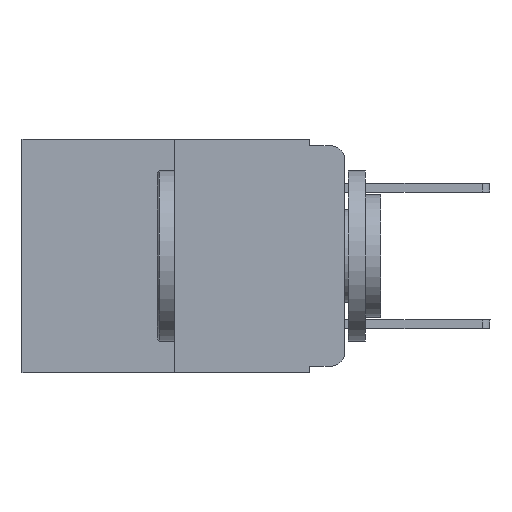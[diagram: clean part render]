
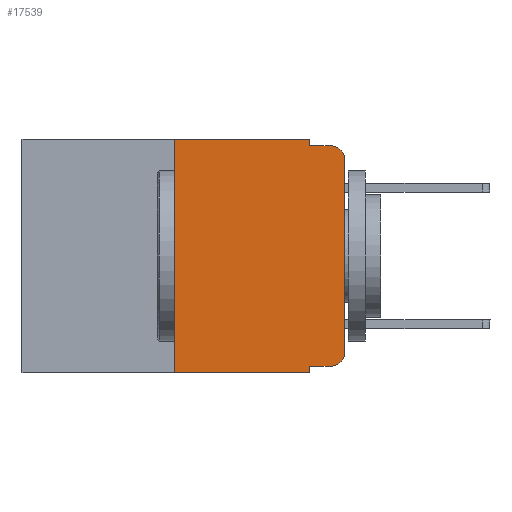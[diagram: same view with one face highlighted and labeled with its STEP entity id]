
A CAD part, left-side view. The second image highlights one B-rep face of the part: STEP entity #17539.
In plain terms, the highlighted planar face has unit normal (-1, 0, 0).
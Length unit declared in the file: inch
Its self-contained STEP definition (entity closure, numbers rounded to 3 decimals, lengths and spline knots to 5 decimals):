
#148 = DIRECTION ( 'NONE',  ( 0., 0., 1. ) ) ;
#819 = CARTESIAN_POINT ( 'NONE',  ( 0., 0.02, -0.333 ) ) ;
#824 = EDGE_CURVE ( 'NONE', #17543, #16498, #5310, .T. ) ;
#1425 = ORIENTED_EDGE ( 'NONE', *, *, #824, .T. ) ;
#1469 = CIRCLE ( 'NONE', #2114, 0.02 ) ;
#1476 = DIRECTION ( 'NONE',  ( 0., -1., 0. ) ) ;
#2114 = AXIS2_PLACEMENT_3D ( 'NONE', #15505, #2840, #5497 ) ;
#2137 = ORIENTED_EDGE ( 'NONE', *, *, #4531, .F. ) ;
#2203 = CARTESIAN_POINT ( 'NONE',  ( 0., 0.051, -0.01 ) ) ;
#2241 = VERTEX_POINT ( 'NONE', #5208 ) ;
#2840 = DIRECTION ( 'NONE',  ( -1., 0., 0. ) ) ;
#3317 = DIRECTION ( 'NONE',  ( 0., 0., -1. ) ) ;
#3366 = DIRECTION ( 'NONE',  ( 0., 0., 1. ) ) ;
#3472 = CARTESIAN_POINT ( 'NONE',  ( 0., 0.051, 0. ) ) ;
#3578 = VERTEX_POINT ( 'NONE', #6424 ) ;
#3598 = CARTESIAN_POINT ( 'NONE',  ( 0., 0.051, 0. ) ) ;
#3768 = VERTEX_POINT ( 'NONE', #4140 ) ;
#3793 = DIRECTION ( 'NONE',  ( 0., 0., -1. ) ) ;
#3851 = DIRECTION ( 'NONE',  ( 0., -1., 0. ) ) ;
#3922 = DIRECTION ( 'NONE',  ( 1., 0., 0. ) ) ;
#4140 = CARTESIAN_POINT ( 'NONE',  ( 0., 0.25, -0.343 ) ) ;
#4506 = VERTEX_POINT ( 'NONE', #819 ) ;
#4531 = EDGE_CURVE ( 'NONE', #5404, #17074, #15727, .T. ) ;
#4542 = CARTESIAN_POINT ( 'NONE',  ( 0., 0.02, -0.01 ) ) ;
#4837 = CIRCLE ( 'NONE', #16959, 0.02 ) ;
#5208 = CARTESIAN_POINT ( 'NONE',  ( 0., 0.051, 0. ) ) ;
#5210 = VECTOR ( 'NONE', #3851, 39.37008 ) ;
#5310 = LINE ( 'NONE', #6305, #10059 ) ;
#5404 = VERTEX_POINT ( 'NONE', #6133 ) ;
#5497 = DIRECTION ( 'NONE',  ( 0., 0., -1. ) ) ;
#5755 = ORIENTED_EDGE ( 'NONE', *, *, #17968, .T. ) ;
#5963 = EDGE_CURVE ( 'NONE', #3578, #2241, #13565, .T. ) ;
#6133 = CARTESIAN_POINT ( 'NONE',  ( 0., 0.051, -0.01 ) ) ;
#6236 = VECTOR ( 'NONE', #1476, 39.37008 ) ;
#6305 = CARTESIAN_POINT ( 'NONE',  ( 0., 0., 0. ) ) ;
#6424 = CARTESIAN_POINT ( 'NONE',  ( 0., 0.25, 0. ) ) ;
#6755 = VECTOR ( 'NONE', #13599, 39.37008 ) ;
#6838 = EDGE_CURVE ( 'NONE', #4506, #17543, #1469, .T. ) ;
#7303 = EDGE_CURVE ( 'NONE', #13460, #17790, #14835, .T. ) ;
#7308 = VECTOR ( 'NONE', #17732, 39.37008 ) ;
#7965 = ORIENTED_EDGE ( 'NONE', *, *, #7303, .F. ) ;
#9004 = CARTESIAN_POINT ( 'NONE',  ( 0., 0.051, -0.343 ) ) ;
#9016 = EDGE_CURVE ( 'NONE', #2241, #5404, #18085, .T. ) ;
#9068 = DIRECTION ( 'NONE',  ( 0., -1., 0. ) ) ;
#9200 = DIRECTION ( 'NONE',  ( -1., 0., 0. ) ) ;
#9745 = CARTESIAN_POINT ( 'NONE',  ( 0., 0., -0.03 ) ) ;
#9868 = CARTESIAN_POINT ( 'NONE',  ( 0., 0.051, -0.333 ) ) ;
#9935 = EDGE_LOOP ( 'NONE', ( #1425, #16983, #2137, #16027, #14566, #16875, #5755, #7965, #12602, #15670 ) ) ;
#10059 = VECTOR ( 'NONE', #3366, 39.37008 ) ;
#10118 = EDGE_CURVE ( 'NONE', #13460, #4506, #14705, .T. ) ;
#10657 = LINE ( 'NONE', #14892, #7308 ) ;
#10706 = DIRECTION ( 'NONE',  ( 0., 0., -1. ) ) ;
#11185 = LINE ( 'NONE', #11563, #12979 ) ;
#11563 = CARTESIAN_POINT ( 'NONE',  ( 0., 0.25, 0. ) ) ;
#12602 = ORIENTED_EDGE ( 'NONE', *, *, #10118, .T. ) ;
#12647 = FACE_OUTER_BOUND ( 'NONE', #9935, .T. ) ;
#12979 = VECTOR ( 'NONE', #148, 39.37008 ) ;
#13362 = CARTESIAN_POINT ( 'NONE',  ( 0., 0.02, -0.03 ) ) ;
#13460 = VERTEX_POINT ( 'NONE', #14985 ) ;
#13565 = LINE ( 'NONE', #14708, #16890 ) ;
#13599 = DIRECTION ( 'NONE',  ( 0., 0., -1. ) ) ;
#13761 = AXIS2_PLACEMENT_3D ( 'NONE', #16762, #3922, #3793 ) ;
#14152 = EDGE_CURVE ( 'NONE', #3768, #3578, #11185, .T. ) ;
#14566 = ORIENTED_EDGE ( 'NONE', *, *, #5963, .F. ) ;
#14705 = LINE ( 'NONE', #9868, #6236 ) ;
#14708 = CARTESIAN_POINT ( 'NONE',  ( 0., 0.473, 0. ) ) ;
#14835 = LINE ( 'NONE', #3598, #15052 ) ;
#14892 = CARTESIAN_POINT ( 'NONE',  ( 0., 0.473, -0.343 ) ) ;
#14985 = CARTESIAN_POINT ( 'NONE',  ( 0., 0.051, -0.333 ) ) ;
#15052 = VECTOR ( 'NONE', #10706, 39.37008 ) ;
#15226 = CARTESIAN_POINT ( 'NONE',  ( 0., 0., -0.313 ) ) ;
#15425 = PLANE ( 'NONE',  #13761 ) ;
#15505 = CARTESIAN_POINT ( 'NONE',  ( 0., 0.02, -0.313 ) ) ;
#15670 = ORIENTED_EDGE ( 'NONE', *, *, #6838, .T. ) ;
#15727 = LINE ( 'NONE', #2203, #5210 ) ;
#16027 = ORIENTED_EDGE ( 'NONE', *, *, #9016, .F. ) ;
#16498 = VERTEX_POINT ( 'NONE', #9745 ) ;
#16762 = CARTESIAN_POINT ( 'NONE',  ( 0., 0.473, 0. ) ) ;
#16875 = ORIENTED_EDGE ( 'NONE', *, *, #14152, .F. ) ;
#16890 = VECTOR ( 'NONE', #9068, 39.37008 ) ;
#16959 = AXIS2_PLACEMENT_3D ( 'NONE', #13362, #9200, #3317 ) ;
#16983 = ORIENTED_EDGE ( 'NONE', *, *, #17297, .T. ) ;
#17074 = VERTEX_POINT ( 'NONE', #4542 ) ;
#17297 = EDGE_CURVE ( 'NONE', #16498, #17074, #4837, .T. ) ;
#17539 = ADVANCED_FACE ( 'NONE', ( #12647 ), #15425, .F. ) ;
#17543 = VERTEX_POINT ( 'NONE', #15226 ) ;
#17732 = DIRECTION ( 'NONE',  ( 0., -1., 0. ) ) ;
#17790 = VERTEX_POINT ( 'NONE', #9004 ) ;
#17968 = EDGE_CURVE ( 'NONE', #3768, #17790, #10657, .T. ) ;
#18085 = LINE ( 'NONE', #3472, #6755 ) ;
